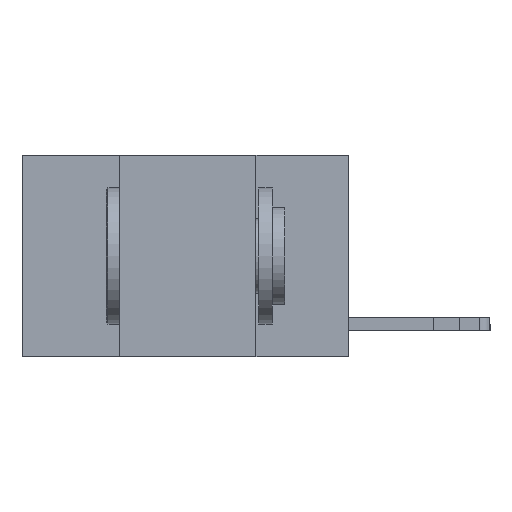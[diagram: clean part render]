
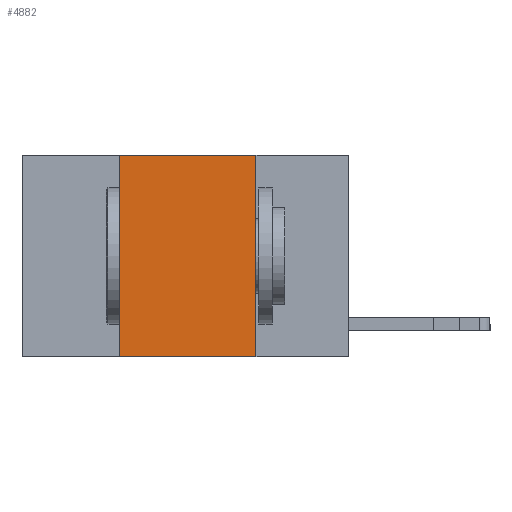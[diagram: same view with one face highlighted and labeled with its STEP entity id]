
A CAD part, left-side view. The second image highlights one B-rep face of the part: STEP entity #4882.
In plain terms, the highlighted planar face has unit normal (-1, 0, 0).
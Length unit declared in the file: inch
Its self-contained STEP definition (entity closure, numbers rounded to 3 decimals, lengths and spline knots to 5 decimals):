
#186 = VERTEX_POINT ( 'NONE', #23311 ) ;
#1341 = EDGE_CURVE ( 'NONE', #186, #15789, #14247, .T. ) ;
#1736 = CARTESIAN_POINT ( 'NONE',  ( 0., 0.6, -0.37 ) ) ;
#3181 = DIRECTION ( 'NONE',  ( 1., 0., 0. ) ) ;
#4882 = ADVANCED_FACE ( 'NONE', ( #14616 ), #5394, .F. ) ;
#5069 = VERTEX_POINT ( 'NONE', #17174 ) ;
#5394 = PLANE ( 'NONE',  #5608 ) ;
#5608 = AXIS2_PLACEMENT_3D ( 'NONE', #22146, #3181, #14862 ) ;
#6001 = CARTESIAN_POINT ( 'NONE',  ( 0., 0.17, -0.37 ) ) ;
#6255 = EDGE_CURVE ( 'NONE', #15789, #5069, #11529, .T. ) ;
#6532 = ORIENTED_EDGE ( 'NONE', *, *, #1341, .F. ) ;
#7315 = LINE ( 'NONE', #14835, #9535 ) ;
#8088 = CARTESIAN_POINT ( 'NONE',  ( 0., 0.6, 0. ) ) ;
#8813 = CARTESIAN_POINT ( 'NONE',  ( 0., 0.42, 0. ) ) ;
#9215 = DIRECTION ( 'NONE',  ( 0., -1., 0. ) ) ;
#9535 = VECTOR ( 'NONE', #22364, 39.37008 ) ;
#11529 = LINE ( 'NONE', #8088, #18353 ) ;
#11660 = EDGE_CURVE ( 'NONE', #186, #21477, #15024, .T. ) ;
#12156 = EDGE_CURVE ( 'NONE', #5069, #21477, #7315, .T. ) ;
#12264 = CARTESIAN_POINT ( 'NONE',  ( 0., 0.42, 0. ) ) ;
#14247 = LINE ( 'NONE', #8813, #16052 ) ;
#14616 = FACE_OUTER_BOUND ( 'NONE', #22805, .T. ) ;
#14835 = CARTESIAN_POINT ( 'NONE',  ( 0., 0.17, 0. ) ) ;
#14843 = ORIENTED_EDGE ( 'NONE', *, *, #11660, .T. ) ;
#14862 = DIRECTION ( 'NONE',  ( 0., 0., -1. ) ) ;
#15024 = LINE ( 'NONE', #1736, #18191 ) ;
#15789 = VERTEX_POINT ( 'NONE', #12264 ) ;
#16052 = VECTOR ( 'NONE', #21783, 39.37008 ) ;
#17174 = CARTESIAN_POINT ( 'NONE',  ( 0., 0.17, 0. ) ) ;
#18191 = VECTOR ( 'NONE', #9215, 39.37008 ) ;
#18353 = VECTOR ( 'NONE', #21044, 39.37008 ) ;
#20232 = ORIENTED_EDGE ( 'NONE', *, *, #12156, .F. ) ;
#21044 = DIRECTION ( 'NONE',  ( 0., -1., 0. ) ) ;
#21477 = VERTEX_POINT ( 'NONE', #6001 ) ;
#21575 = ORIENTED_EDGE ( 'NONE', *, *, #6255, .F. ) ;
#21783 = DIRECTION ( 'NONE',  ( 0., 0., 1. ) ) ;
#22146 = CARTESIAN_POINT ( 'NONE',  ( 0., 0.6, 0. ) ) ;
#22364 = DIRECTION ( 'NONE',  ( 0., 0., -1. ) ) ;
#22805 = EDGE_LOOP ( 'NONE', ( #20232, #21575, #6532, #14843 ) ) ;
#23311 = CARTESIAN_POINT ( 'NONE',  ( 0., 0.42, -0.37 ) ) ;
